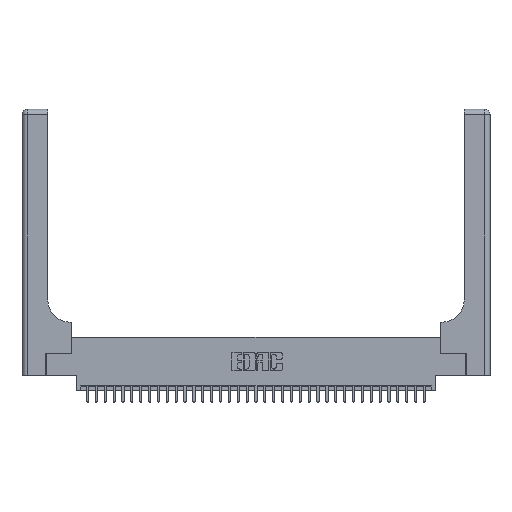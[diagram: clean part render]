
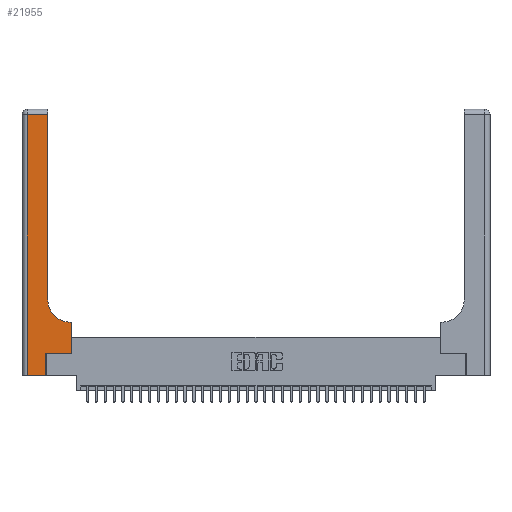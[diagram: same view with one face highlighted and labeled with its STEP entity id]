
A CAD part, top view. The second image highlights one B-rep face of the part: STEP entity #21955.
In plain terms, the highlighted planar face has unit normal (0, 0, 1).
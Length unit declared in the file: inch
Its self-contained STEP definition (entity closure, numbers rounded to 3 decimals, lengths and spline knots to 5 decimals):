
#218 = CARTESIAN_POINT ( 'NONE',  ( 0., 0., 0.37 ) ) ;
#321 = DIRECTION ( 'NONE',  ( 1., 0., 0. ) ) ;
#405 = VECTOR ( 'NONE', #34777, 39.37008 ) ;
#431 = CARTESIAN_POINT ( 'NONE',  ( 0.5585, 0.25, 0.37 ) ) ;
#660 = CARTESIAN_POINT ( 'NONE',  ( 0.5415, 0.85, 0.37 ) ) ;
#2071 = VECTOR ( 'NONE', #25451, 39.37008 ) ;
#2409 = VERTEX_POINT ( 'NONE', #19005 ) ;
#2436 = CARTESIAN_POINT ( 'NONE',  ( 0.06, 0., 0.37 ) ) ;
#2716 = CARTESIAN_POINT ( 'NONE',  ( 0.06, 2.94, 0.37 ) ) ;
#3112 = ORIENTED_EDGE ( 'NONE', *, *, #34516, .T. ) ;
#3232 = VECTOR ( 'NONE', #18968, 39.37008 ) ;
#3489 = DIRECTION ( 'NONE',  ( 0., 0., -1. ) ) ;
#4738 = LINE ( 'NONE', #35959, #27943 ) ;
#5464 = DIRECTION ( 'NONE',  ( 0., 0., -1. ) ) ;
#6334 = CARTESIAN_POINT ( 'NONE',  ( 0.5585, 0.6, 0.37 ) ) ;
#6593 = CARTESIAN_POINT ( 'NONE',  ( 0.2915, 3., 0.37 ) ) ;
#7032 = LINE ( 'NONE', #6593, #405 ) ;
#7236 = LINE ( 'NONE', #30638, #20761 ) ;
#7612 = CARTESIAN_POINT ( 'NONE',  ( 0.269, 0.25, 0.37 ) ) ;
#7730 = DIRECTION ( 'NONE',  ( -1., 0., 0. ) ) ;
#7847 = ORIENTED_EDGE ( 'NONE', *, *, #21311, .T. ) ;
#7914 = DIRECTION ( 'NONE',  ( -1., 0., 0. ) ) ;
#8037 = PLANE ( 'NONE',  #29626 ) ;
#8124 = VERTEX_POINT ( 'NONE', #2716 ) ;
#9573 = LINE ( 'NONE', #218, #22699 ) ;
#10131 = VERTEX_POINT ( 'NONE', #12860 ) ;
#10550 = ORIENTED_EDGE ( 'NONE', *, *, #26599, .T. ) ;
#11000 = VERTEX_POINT ( 'NONE', #28795 ) ;
#11575 = VERTEX_POINT ( 'NONE', #2436 ) ;
#11696 = ORIENTED_EDGE ( 'NONE', *, *, #13337, .T. ) ;
#11933 = DIRECTION ( 'NONE',  ( 1., 0., 0. ) ) ;
#12237 = FACE_OUTER_BOUND ( 'NONE', #12458, .T. ) ;
#12431 = CARTESIAN_POINT ( 'NONE',  ( 0.06, 3., 0.37 ) ) ;
#12458 = EDGE_LOOP ( 'NONE', ( #7847, #15769, #10550, #32789, #11696, #14373, #3112, #24224, #27091 ) ) ;
#12860 = CARTESIAN_POINT ( 'NONE',  ( 0.2915, 0.85, 0.37 ) ) ;
#13337 = EDGE_CURVE ( 'NONE', #18878, #11000, #32257, .T. ) ;
#14373 = ORIENTED_EDGE ( 'NONE', *, *, #36105, .T. ) ;
#14697 = DIRECTION ( 'NONE',  ( 0., 1., 0. ) ) ;
#15075 = EDGE_CURVE ( 'NONE', #17037, #2409, #4738, .T. ) ;
#15400 = DIRECTION ( 'NONE',  ( 0., -1., 0. ) ) ;
#15762 = CARTESIAN_POINT ( 'NONE',  ( 0.269, 0., 0.37 ) ) ;
#15769 = ORIENTED_EDGE ( 'NONE', *, *, #33289, .T. ) ;
#17037 = VERTEX_POINT ( 'NONE', #6334 ) ;
#17500 = CARTESIAN_POINT ( 'NONE',  ( 0.5585, 0.25, 0.37 ) ) ;
#17770 = VECTOR ( 'NONE', #14697, 39.37008 ) ;
#18878 = VERTEX_POINT ( 'NONE', #15762 ) ;
#18968 = DIRECTION ( 'NONE',  ( 1., 0., 0. ) ) ;
#19005 = CARTESIAN_POINT ( 'NONE',  ( 0.5415, 0.6, 0.37 ) ) ;
#19553 = CIRCLE ( 'NONE', #35736, 0.25 ) ;
#20586 = VERTEX_POINT ( 'NONE', #17500 ) ;
#20761 = VECTOR ( 'NONE', #27710, 39.37008 ) ;
#21311 = EDGE_CURVE ( 'NONE', #10131, #24989, #7032, .T. ) ;
#21955 = ADVANCED_FACE ( 'NONE', ( #12237 ), #8037, .F. ) ;
#22630 = EDGE_CURVE ( 'NONE', #11575, #18878, #9573, .T. ) ;
#22699 = VECTOR ( 'NONE', #321, 39.37008 ) ;
#24224 = ORIENTED_EDGE ( 'NONE', *, *, #15075, .T. ) ;
#24426 = CARTESIAN_POINT ( 'NONE',  ( 0.269, 0., 0.37 ) ) ;
#24686 = EDGE_CURVE ( 'NONE', #2409, #10131, #19553, .T. ) ;
#24989 = VERTEX_POINT ( 'NONE', #33148 ) ;
#25451 = DIRECTION ( 'NONE',  ( 0., 1., 0. ) ) ;
#25917 = VECTOR ( 'NONE', #15400, 39.37008 ) ;
#26599 = EDGE_CURVE ( 'NONE', #8124, #11575, #33852, .T. ) ;
#27091 = ORIENTED_EDGE ( 'NONE', *, *, #24686, .T. ) ;
#27710 = DIRECTION ( 'NONE',  ( -1., 0., 0. ) ) ;
#27943 = VECTOR ( 'NONE', #7730, 39.37008 ) ;
#28305 = LINE ( 'NONE', #431, #2071 ) ;
#28795 = CARTESIAN_POINT ( 'NONE',  ( 0.269, 0.25, 0.37 ) ) ;
#29626 = AXIS2_PLACEMENT_3D ( 'NONE', #30195, #5464, #7914 ) ;
#30195 = CARTESIAN_POINT ( 'NONE',  ( 0., 3., 0.37 ) ) ;
#30638 = CARTESIAN_POINT ( 'NONE',  ( 0., 2.94, 0.37 ) ) ;
#32257 = LINE ( 'NONE', #24426, #17770 ) ;
#32789 = ORIENTED_EDGE ( 'NONE', *, *, #22630, .T. ) ;
#33148 = CARTESIAN_POINT ( 'NONE',  ( 0.2915, 2.94, 0.37 ) ) ;
#33289 = EDGE_CURVE ( 'NONE', #24989, #8124, #7236, .T. ) ;
#33852 = LINE ( 'NONE', #12431, #25917 ) ;
#34368 = LINE ( 'NONE', #7612, #3232 ) ;
#34516 = EDGE_CURVE ( 'NONE', #20586, #17037, #28305, .T. ) ;
#34777 = DIRECTION ( 'NONE',  ( 0., 1., 0. ) ) ;
#35736 = AXIS2_PLACEMENT_3D ( 'NONE', #660, #3489, #11933 ) ;
#35959 = CARTESIAN_POINT ( 'NONE',  ( 0.2915, 0.6, 0.37 ) ) ;
#36105 = EDGE_CURVE ( 'NONE', #11000, #20586, #34368, .T. ) ;
